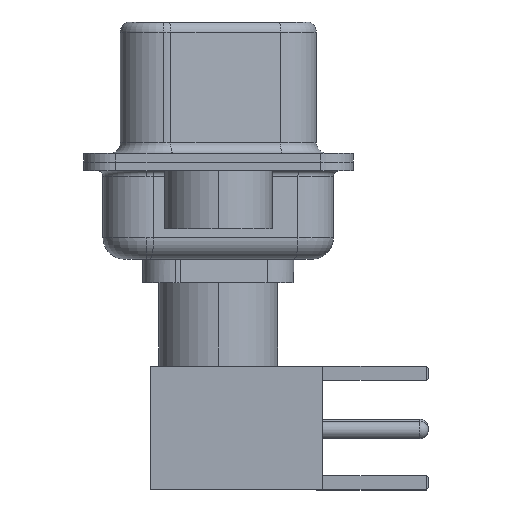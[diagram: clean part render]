
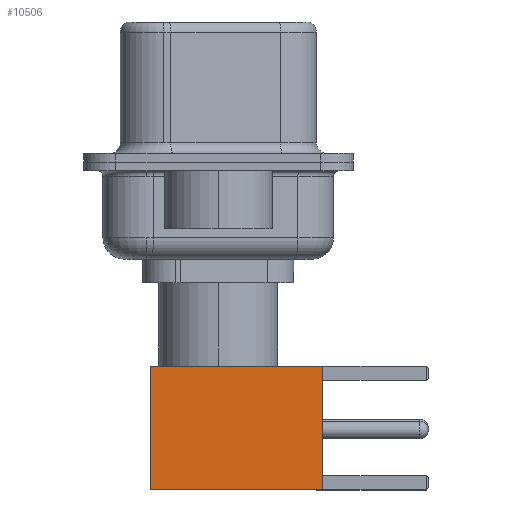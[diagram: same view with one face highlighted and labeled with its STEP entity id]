
A CAD part, left-side view. The second image highlights one B-rep face of the part: STEP entity #10506.
In plain terms, the highlighted face is planar.
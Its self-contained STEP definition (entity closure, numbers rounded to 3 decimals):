
#107 = DIRECTION ( 'NONE',  ( 0., 1., 0. ) ) ;
#171 = LINE ( 'NONE', #17982, #10533 ) ;
#203 = ORIENTED_EDGE ( 'NONE', *, *, #7537, .T. ) ;
#242 = CARTESIAN_POINT ( 'NONE',  ( 2.875, 2.875, 0. ) ) ;
#435 = CARTESIAN_POINT ( 'NONE',  ( 2.875, 2.875, 8. ) ) ;
#596 = CARTESIAN_POINT ( 'NONE',  ( -2.875, 2.875, 0. ) ) ;
#690 = ORIENTED_EDGE ( 'NONE', *, *, #1887, .T. ) ;
#706 = CARTESIAN_POINT ( 'NONE',  ( -2.875, 2.875, 8. ) ) ;
#1116 = VECTOR ( 'NONE', #6426, 1000. ) ;
#1586 = PLANE ( 'NONE',  #11842 ) ;
#1676 = CARTESIAN_POINT ( 'NONE',  ( 0., 2.875, 8. ) ) ;
#1887 = EDGE_CURVE ( 'NONE', #17172, #2699, #15141, .T. ) ;
#2536 = ORIENTED_EDGE ( 'NONE', *, *, #7309, .F. ) ;
#2699 = VERTEX_POINT ( 'NONE', #8725 ) ;
#3371 = LINE ( 'NONE', #1676, #4604 ) ;
#4604 = VECTOR ( 'NONE', #15508, 1000. ) ;
#6060 = CARTESIAN_POINT ( 'NONE',  ( 0., 2.875, 0. ) ) ;
#6231 = EDGE_LOOP ( 'NONE', ( #203, #690, #2536, #7064 ) ) ;
#6350 = VERTEX_POINT ( 'NONE', #435 ) ;
#6426 = DIRECTION ( 'NONE',  ( 0., 0., -1. ) ) ;
#6824 = VERTEX_POINT ( 'NONE', #706 ) ;
#7064 = ORIENTED_EDGE ( 'NONE', *, *, #10733, .F. ) ;
#7309 = EDGE_CURVE ( 'NONE', #6824, #2699, #7901, .T. ) ;
#7537 = EDGE_CURVE ( 'NONE', #6350, #17172, #171, .T. ) ;
#7901 = LINE ( 'NONE', #596, #1116 ) ;
#8725 = CARTESIAN_POINT ( 'NONE',  ( -2.875, 2.875, 0. ) ) ;
#9012 = CARTESIAN_POINT ( 'NONE',  ( 2.875, 2.875, 0. ) ) ;
#10506 = ADVANCED_FACE ( 'NONE', ( #18099 ), #1586, .T. ) ;
#10533 = VECTOR ( 'NONE', #19353, 1000. ) ;
#10689 = DIRECTION ( 'NONE',  ( 0., 0., 1. ) ) ;
#10733 = EDGE_CURVE ( 'NONE', #6350, #6824, #3371, .T. ) ;
#11842 = AXIS2_PLACEMENT_3D ( 'NONE', #9012, #107, #10689 ) ;
#13366 = VECTOR ( 'NONE', #16433, 1000. ) ;
#15141 = LINE ( 'NONE', #6060, #13366 ) ;
#15508 = DIRECTION ( 'NONE',  ( -1., 0., 0. ) ) ;
#16433 = DIRECTION ( 'NONE',  ( -1., 0., 0. ) ) ;
#17172 = VERTEX_POINT ( 'NONE', #242 ) ;
#17982 = CARTESIAN_POINT ( 'NONE',  ( 2.875, 2.875, 0. ) ) ;
#18099 = FACE_OUTER_BOUND ( 'NONE', #6231, .T. ) ;
#19353 = DIRECTION ( 'NONE',  ( 0., 0., -1. ) ) ;
